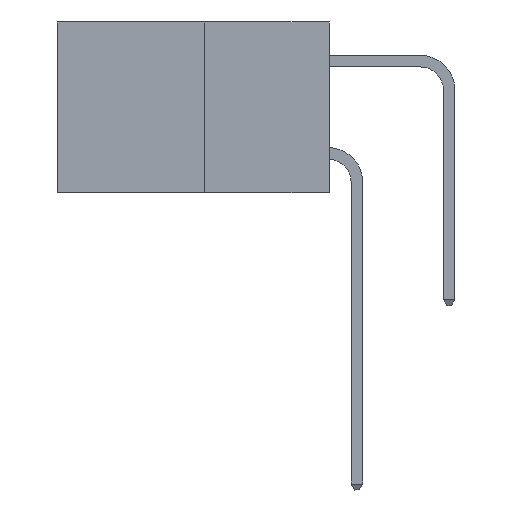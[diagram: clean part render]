
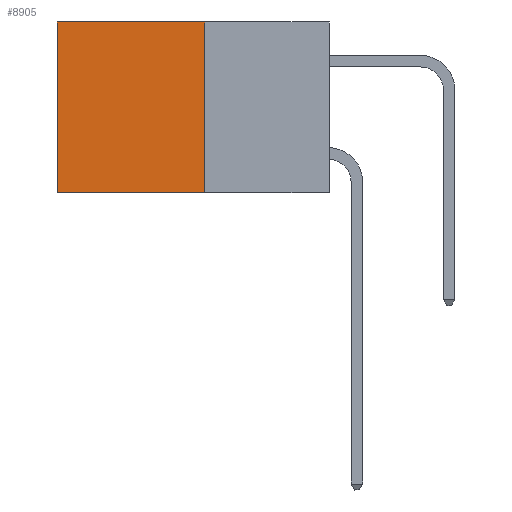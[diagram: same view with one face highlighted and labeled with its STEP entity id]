
A CAD part, left-side view. The second image highlights one B-rep face of the part: STEP entity #8905.
In plain terms, the highlighted planar face has unit normal (-1, 0, 0).
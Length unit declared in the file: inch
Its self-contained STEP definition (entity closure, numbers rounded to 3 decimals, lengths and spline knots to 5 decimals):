
#122 = VERTEX_POINT ( 'NONE', #7574 ) ;
#1156 = FACE_OUTER_BOUND ( 'NONE', #2711, .T. ) ;
#1491 = VERTEX_POINT ( 'NONE', #1859 ) ;
#1859 = CARTESIAN_POINT ( 'NONE',  ( 0.277, 0.27, 0. ) ) ;
#2429 = DIRECTION ( 'NONE',  ( 0., 0., -1. ) ) ;
#2711 = EDGE_LOOP ( 'NONE', ( #3913, #5542, #3837, #11599 ) ) ;
#3192 = CARTESIAN_POINT ( 'NONE',  ( 0.277, 0.27, -0.37 ) ) ;
#3283 = VERTEX_POINT ( 'NONE', #6854 ) ;
#3317 = PLANE ( 'NONE',  #10209 ) ;
#3582 = DIRECTION ( 'NONE',  ( 0., 0., -1. ) ) ;
#3625 = EDGE_CURVE ( 'NONE', #1491, #3283, #7478, .T. ) ;
#3837 = ORIENTED_EDGE ( 'NONE', *, *, #3625, .F. ) ;
#3913 = ORIENTED_EDGE ( 'NONE', *, *, #10893, .T. ) ;
#4979 = VECTOR ( 'NONE', #2429, 39.37008 ) ;
#5242 = DIRECTION ( 'NONE',  ( 1., 0., 0. ) ) ;
#5276 = CARTESIAN_POINT ( 'NONE',  ( 0.277, 0.27, -0.37 ) ) ;
#5280 = LINE ( 'NONE', #6612, #11879 ) ;
#5534 = EDGE_CURVE ( 'NONE', #3283, #7250, #8931, .T. ) ;
#5542 = ORIENTED_EDGE ( 'NONE', *, *, #5534, .F. ) ;
#6019 = DIRECTION ( 'NONE',  ( 0., 1., 0. ) ) ;
#6143 = CARTESIAN_POINT ( 'NONE',  ( 0.277, 0.27, -0.37 ) ) ;
#6612 = CARTESIAN_POINT ( 'NONE',  ( 0.277, 0.27, 0. ) ) ;
#6854 = CARTESIAN_POINT ( 'NONE',  ( 0.277, 0.27, -0.37 ) ) ;
#7250 = VERTEX_POINT ( 'NONE', #11584 ) ;
#7478 = LINE ( 'NONE', #5276, #4979 ) ;
#7574 = CARTESIAN_POINT ( 'NONE',  ( 0.277, 0.59, 0. ) ) ;
#8355 = CARTESIAN_POINT ( 'NONE',  ( 0.277, 0.59, -0.37 ) ) ;
#8511 = DIRECTION ( 'NONE',  ( 0., 1., 0. ) ) ;
#8543 = EDGE_CURVE ( 'NONE', #1491, #122, #5280, .T. ) ;
#8905 = ADVANCED_FACE ( 'NONE', ( #1156 ), #3317, .F. ) ;
#8931 = LINE ( 'NONE', #3192, #11108 ) ;
#9887 = VECTOR ( 'NONE', #3582, 39.37008 ) ;
#10178 = LINE ( 'NONE', #8355, #9887 ) ;
#10209 = AXIS2_PLACEMENT_3D ( 'NONE', #6143, #5242, #11813 ) ;
#10893 = EDGE_CURVE ( 'NONE', #122, #7250, #10178, .T. ) ;
#11108 = VECTOR ( 'NONE', #6019, 39.37008 ) ;
#11584 = CARTESIAN_POINT ( 'NONE',  ( 0.277, 0.59, -0.37 ) ) ;
#11599 = ORIENTED_EDGE ( 'NONE', *, *, #8543, .T. ) ;
#11813 = DIRECTION ( 'NONE',  ( 0., 0., -1. ) ) ;
#11879 = VECTOR ( 'NONE', #8511, 39.37008 ) ;
